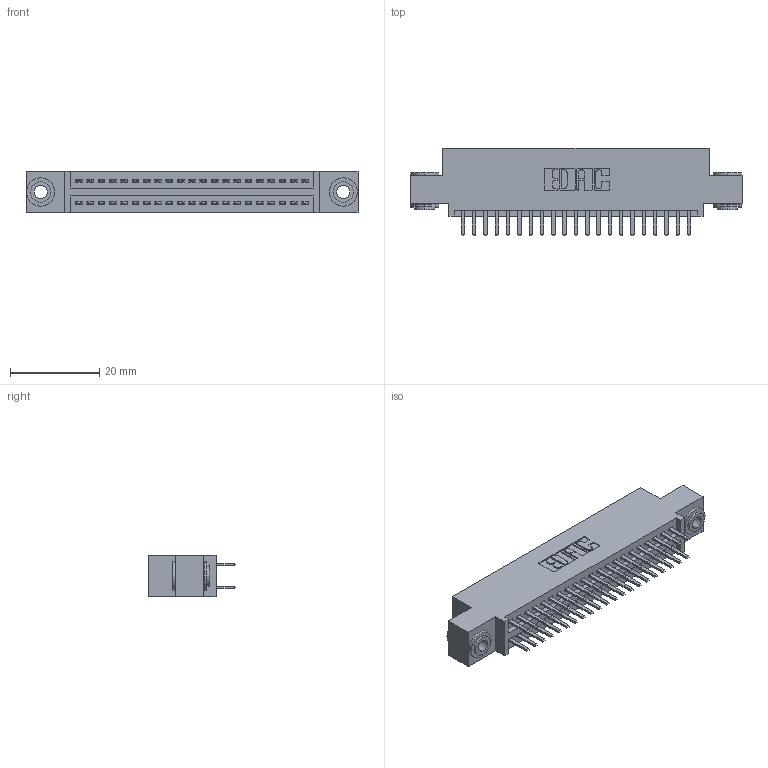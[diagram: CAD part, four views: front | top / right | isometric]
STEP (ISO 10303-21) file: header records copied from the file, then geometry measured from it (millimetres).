
FILE_DESCRIPTION (( 'STEP AP203' ), '1' );
FILE_NAME ('395-042-520-503.STEP', '2018-11-15T07:32:37', ( '' ), ( '' ), 'SwSTEP 2.0', 'SolidWorks 2016', '' );
FILE_SCHEMA (( 'CONFIG_CONTROL_DESIGN' ));
Length unit declared in the file: inch
Products named in the file (4): 395-042-520-503; 345 Part_0.110 Offset - 0.156 Dia-TH; 345-292-001_345-293-120; 345-250-002_345-250-002-102
Assembly tree (45 placements, depth 2):
  395-042-520-503
    345 Part_0.110 Offset - 0.156 Dia-TH
    345-292-001_345-293-120  x42
    345-250-002_345-250-002-102  x2
Bounding box: 74.55 x 19.68 x 9.4 mm (x, y, z)
Volume: 6974.4 mm3; surface area: 10161.1 mm2
Topology: 45 solids, 45 shells, 2436 faces, 7023 edges, 4566 vertices
Faces by surface type: plane 1564, cylinder 864, cone 8
Entity records: 20200 total; most frequent: CARTESIAN_POINT 3395, ORIENTED_EDGE 3310, DIRECTION 3037, EDGE_CURVE 1655, LINE 1411, VECTOR 1411, VERTEX_POINT 1098, AXIS2_PLACEMENT_3D 813
